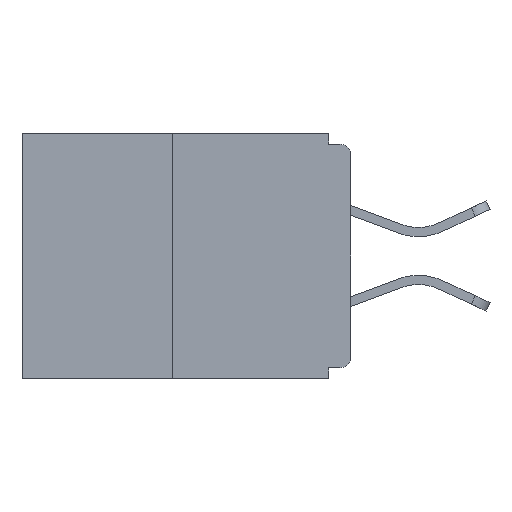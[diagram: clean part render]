
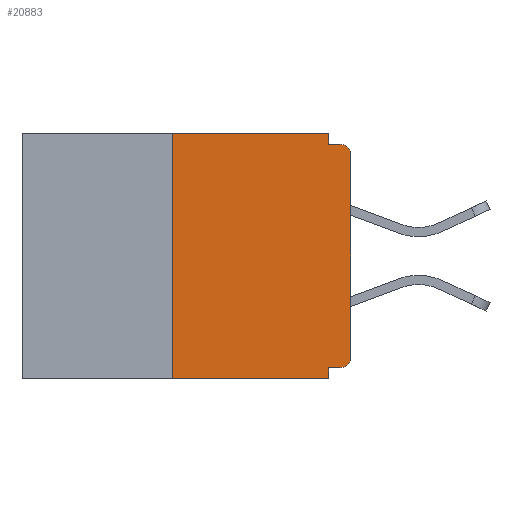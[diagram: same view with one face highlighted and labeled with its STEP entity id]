
A CAD part, left-side view. The second image highlights one B-rep face of the part: STEP entity #20883.
In plain terms, the highlighted planar face has unit normal (-1, 0, 0).
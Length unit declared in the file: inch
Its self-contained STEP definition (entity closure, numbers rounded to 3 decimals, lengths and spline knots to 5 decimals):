
#596 = VECTOR ( 'NONE', #13752, 39.37008 ) ;
#663 = LINE ( 'NONE', #6732, #9316 ) ;
#746 = LINE ( 'NONE', #15285, #14117 ) ;
#1320 = CARTESIAN_POINT ( 'NONE',  ( 0., 0.031, -0.343 ) ) ;
#1466 = DIRECTION ( 'NONE',  ( 0., 0., 1. ) ) ;
#1856 = CARTESIAN_POINT ( 'NONE',  ( 0., 0.031, -0.015 ) ) ;
#2179 = ORIENTED_EDGE ( 'NONE', *, *, #7547, .T. ) ;
#2204 = ORIENTED_EDGE ( 'NONE', *, *, #2761, .F. ) ;
#2743 = CARTESIAN_POINT ( 'NONE',  ( 0., 0.25, -0.343 ) ) ;
#2761 = EDGE_CURVE ( 'NONE', #17995, #21540, #4641, .T. ) ;
#3064 = EDGE_CURVE ( 'NONE', #5232, #5012, #13967, .T. ) ;
#3082 = LINE ( 'NONE', #22872, #17078 ) ;
#3172 = PLANE ( 'NONE',  #13267 ) ;
#4641 = LINE ( 'NONE', #12428, #4940 ) ;
#4940 = VECTOR ( 'NONE', #8587, 39.37008 ) ;
#5012 = VERTEX_POINT ( 'NONE', #7485 ) ;
#5232 = VERTEX_POINT ( 'NONE', #24885 ) ;
#6134 = CARTESIAN_POINT ( 'NONE',  ( 0., 0., -0.03 ) ) ;
#6310 = ORIENTED_EDGE ( 'NONE', *, *, #3064, .F. ) ;
#6732 = CARTESIAN_POINT ( 'NONE',  ( 0., 0.031, 0. ) ) ;
#6792 = EDGE_LOOP ( 'NONE', ( #9591, #20090, #13975, #6310, #9808, #20725, #9452, #2179, #2204, #17805 ) ) ;
#6927 = AXIS2_PLACEMENT_3D ( 'NONE', #13346, #15264, #13172 ) ;
#7230 = DIRECTION ( 'NONE',  ( 0., 0., -1. ) ) ;
#7279 = CARTESIAN_POINT ( 'NONE',  ( 0., 0.46, -0.343 ) ) ;
#7485 = CARTESIAN_POINT ( 'NONE',  ( 0., 0.031, -0.343 ) ) ;
#7547 = EDGE_CURVE ( 'NONE', #18388, #21540, #17874, .T. ) ;
#7785 = DIRECTION ( 'NONE',  ( -1., 0., 0. ) ) ;
#8248 = VECTOR ( 'NONE', #23284, 39.37008 ) ;
#8587 = DIRECTION ( 'NONE',  ( 0., -1., 0. ) ) ;
#9157 = EDGE_CURVE ( 'NONE', #25583, #17995, #663, .T. ) ;
#9264 = DIRECTION ( 'NONE',  ( 0., 1., 0. ) ) ;
#9311 = VERTEX_POINT ( 'NONE', #13006 ) ;
#9316 = VECTOR ( 'NONE', #24839, 39.37008 ) ;
#9398 = DIRECTION ( 'NONE',  ( 0., 0., 1. ) ) ;
#9452 = ORIENTED_EDGE ( 'NONE', *, *, #14844, .T. ) ;
#9591 = ORIENTED_EDGE ( 'NONE', *, *, #21225, .F. ) ;
#9808 = ORIENTED_EDGE ( 'NONE', *, *, #10936, .F. ) ;
#10265 = AXIS2_PLACEMENT_3D ( 'NONE', #17532, #7785, #13797 ) ;
#10936 = EDGE_CURVE ( 'NONE', #9311, #5232, #3082, .T. ) ;
#11050 = CIRCLE ( 'NONE', #10265, 0.015 ) ;
#11368 = LINE ( 'NONE', #19071, #17304 ) ;
#11682 = LINE ( 'NONE', #7279, #8248 ) ;
#11971 = FACE_OUTER_BOUND ( 'NONE', #6792, .T. ) ;
#12428 = CARTESIAN_POINT ( 'NONE',  ( 0., 0., -0.015 ) ) ;
#12818 = EDGE_CURVE ( 'NONE', #9311, #17551, #11050, .T. ) ;
#12871 = CARTESIAN_POINT ( 'NONE',  ( 0., 0.031, 0. ) ) ;
#13006 = CARTESIAN_POINT ( 'NONE',  ( 0., 0.015, -0.328 ) ) ;
#13172 = DIRECTION ( 'NONE',  ( 0., 0., -1. ) ) ;
#13267 = AXIS2_PLACEMENT_3D ( 'NONE', #21088, #19180, #7230 ) ;
#13346 = CARTESIAN_POINT ( 'NONE',  ( 0., 0.015, -0.03 ) ) ;
#13752 = DIRECTION ( 'NONE',  ( 0., 0., -1. ) ) ;
#13769 = EDGE_CURVE ( 'NONE', #18671, #5012, #11682, .T. ) ;
#13797 = DIRECTION ( 'NONE',  ( 0., 0., -1. ) ) ;
#13967 = LINE ( 'NONE', #1320, #596 ) ;
#13975 = ORIENTED_EDGE ( 'NONE', *, *, #13769, .T. ) ;
#14117 = VECTOR ( 'NONE', #1466, 39.37008 ) ;
#14177 = LINE ( 'NONE', #17355, #24131 ) ;
#14844 = EDGE_CURVE ( 'NONE', #17551, #18388, #14177, .T. ) ;
#15264 = DIRECTION ( 'NONE',  ( -1., 0., 0. ) ) ;
#15285 = CARTESIAN_POINT ( 'NONE',  ( 0., 0.25, 0. ) ) ;
#15493 = CARTESIAN_POINT ( 'NONE',  ( 0., 0.25, 0. ) ) ;
#16682 = CARTESIAN_POINT ( 'NONE',  ( 0., 0., -0.313 ) ) ;
#17078 = VECTOR ( 'NONE', #9264, 39.37008 ) ;
#17304 = VECTOR ( 'NONE', #21400, 39.37008 ) ;
#17355 = CARTESIAN_POINT ( 'NONE',  ( 0., 0., 0. ) ) ;
#17532 = CARTESIAN_POINT ( 'NONE',  ( 0., 0.015, -0.313 ) ) ;
#17551 = VERTEX_POINT ( 'NONE', #16682 ) ;
#17805 = ORIENTED_EDGE ( 'NONE', *, *, #9157, .F. ) ;
#17874 = CIRCLE ( 'NONE', #6927, 0.015 ) ;
#17995 = VERTEX_POINT ( 'NONE', #1856 ) ;
#18388 = VERTEX_POINT ( 'NONE', #6134 ) ;
#18671 = VERTEX_POINT ( 'NONE', #2743 ) ;
#19071 = CARTESIAN_POINT ( 'NONE',  ( 0., 0.46, 0. ) ) ;
#19180 = DIRECTION ( 'NONE',  ( 1., 0., 0. ) ) ;
#20090 = ORIENTED_EDGE ( 'NONE', *, *, #22682, .F. ) ;
#20725 = ORIENTED_EDGE ( 'NONE', *, *, #12818, .T. ) ;
#20748 = CARTESIAN_POINT ( 'NONE',  ( 0., 0.015, -0.015 ) ) ;
#20883 = ADVANCED_FACE ( 'NONE', ( #11971 ), #3172, .F. ) ;
#21088 = CARTESIAN_POINT ( 'NONE',  ( 0., 0.46, 0. ) ) ;
#21225 = EDGE_CURVE ( 'NONE', #21303, #25583, #11368, .T. ) ;
#21303 = VERTEX_POINT ( 'NONE', #15493 ) ;
#21400 = DIRECTION ( 'NONE',  ( 0., -1., 0. ) ) ;
#21540 = VERTEX_POINT ( 'NONE', #20748 ) ;
#22682 = EDGE_CURVE ( 'NONE', #18671, #21303, #746, .T. ) ;
#22872 = CARTESIAN_POINT ( 'NONE',  ( 0., 0., -0.328 ) ) ;
#23284 = DIRECTION ( 'NONE',  ( 0., -1., 0. ) ) ;
#24131 = VECTOR ( 'NONE', #9398, 39.37008 ) ;
#24839 = DIRECTION ( 'NONE',  ( 0., 0., -1. ) ) ;
#24885 = CARTESIAN_POINT ( 'NONE',  ( 0., 0.031, -0.328 ) ) ;
#25583 = VERTEX_POINT ( 'NONE', #12871 ) ;
